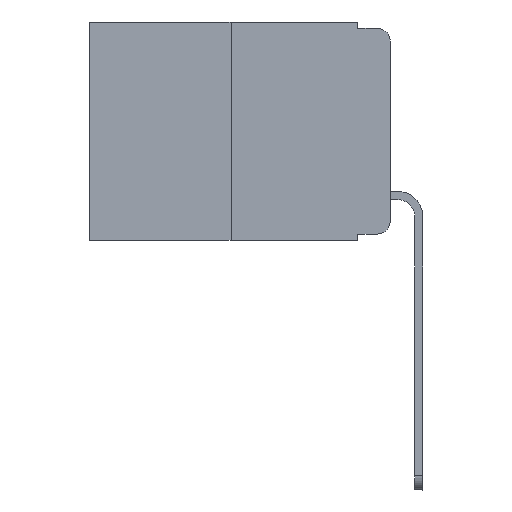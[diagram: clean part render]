
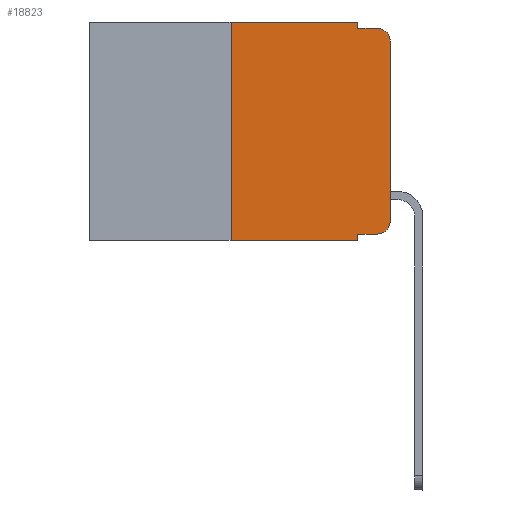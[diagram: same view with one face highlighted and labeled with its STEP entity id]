
A CAD part, left-side view. The second image highlights one B-rep face of the part: STEP entity #18823.
In plain terms, the highlighted planar face has unit normal (-1, 0, 0).
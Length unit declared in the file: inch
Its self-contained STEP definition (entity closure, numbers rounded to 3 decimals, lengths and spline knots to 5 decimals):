
#326 = EDGE_CURVE ( 'NONE', #14275, #2661, #22049, .T. ) ;
#783 = LINE ( 'NONE', #25401, #3292 ) ;
#1665 = VECTOR ( 'NONE', #16096, 39.37008 ) ;
#2250 = VECTOR ( 'NONE', #9095, 39.37008 ) ;
#2661 = VERTEX_POINT ( 'NONE', #17127 ) ;
#2748 = CARTESIAN_POINT ( 'NONE',  ( 0., 0.25, 0. ) ) ;
#2987 = ORIENTED_EDGE ( 'NONE', *, *, #16214, .T. ) ;
#3099 = ORIENTED_EDGE ( 'NONE', *, *, #326, .F. ) ;
#3292 = VECTOR ( 'NONE', #9144, 39.37008 ) ;
#3828 = EDGE_CURVE ( 'NONE', #10233, #14029, #17336, .T. ) ;
#3970 = CARTESIAN_POINT ( 'NONE',  ( 0., 0.02, -0.03 ) ) ;
#4244 = VECTOR ( 'NONE', #16767, 39.37008 ) ;
#4571 = LINE ( 'NONE', #13319, #2250 ) ;
#4583 = DIRECTION ( 'NONE',  ( 1., 0., 0. ) ) ;
#4977 = VERTEX_POINT ( 'NONE', #24141 ) ;
#5129 = DIRECTION ( 'NONE',  ( 0., 0., 1. ) ) ;
#5194 = CIRCLE ( 'NONE', #20494, 0.02 ) ;
#6585 = VERTEX_POINT ( 'NONE', #20843 ) ;
#6778 = CARTESIAN_POINT ( 'NONE',  ( 0., 0.25, 0. ) ) ;
#6905 = CARTESIAN_POINT ( 'NONE',  ( 0., 0.473, 0. ) ) ;
#6907 = LINE ( 'NONE', #6778, #19446 ) ;
#7227 = EDGE_LOOP ( 'NONE', ( #26319, #15640, #26040, #3099, #22942, #13227, #10855, #12541, #2987, #14217 ) ) ;
#7603 = DIRECTION ( 'NONE',  ( 0., 0., -1. ) ) ;
#7754 = CARTESIAN_POINT ( 'NONE',  ( 0., 0., 0. ) ) ;
#8421 = CARTESIAN_POINT ( 'NONE',  ( 0., 0.473, -0.343 ) ) ;
#8543 = VECTOR ( 'NONE', #18561, 39.37008 ) ;
#8771 = CARTESIAN_POINT ( 'NONE',  ( 0., 0.051, 0. ) ) ;
#9095 = DIRECTION ( 'NONE',  ( 0., 0., -1. ) ) ;
#9144 = DIRECTION ( 'NONE',  ( 0., -1., 0. ) ) ;
#9591 = DIRECTION ( 'NONE',  ( 0., 0., -1. ) ) ;
#10212 = VERTEX_POINT ( 'NONE', #18459 ) ;
#10233 = VERTEX_POINT ( 'NONE', #26485 ) ;
#10532 = EDGE_CURVE ( 'NONE', #11421, #14275, #783, .T. ) ;
#10855 = ORIENTED_EDGE ( 'NONE', *, *, #17451, .T. ) ;
#10872 = PLANE ( 'NONE',  #22212 ) ;
#11386 = CARTESIAN_POINT ( 'NONE',  ( 0., 0.051, 0. ) ) ;
#11421 = VERTEX_POINT ( 'NONE', #2748 ) ;
#11928 = EDGE_CURVE ( 'NONE', #14029, #21160, #26198, .T. ) ;
#12328 = DIRECTION ( 'NONE',  ( -1., 0., 0. ) ) ;
#12541 = ORIENTED_EDGE ( 'NONE', *, *, #23210, .F. ) ;
#12907 = LINE ( 'NONE', #25079, #26663 ) ;
#13227 = ORIENTED_EDGE ( 'NONE', *, *, #13306, .F. ) ;
#13306 = EDGE_CURVE ( 'NONE', #4977, #11421, #6907, .T. ) ;
#13319 = CARTESIAN_POINT ( 'NONE',  ( 0., 0.051, 0. ) ) ;
#13845 = VERTEX_POINT ( 'NONE', #19761 ) ;
#14029 = VERTEX_POINT ( 'NONE', #22983 ) ;
#14145 = DIRECTION ( 'NONE',  ( -1., 0., 0. ) ) ;
#14217 = ORIENTED_EDGE ( 'NONE', *, *, #3828, .T. ) ;
#14275 = VERTEX_POINT ( 'NONE', #8771 ) ;
#14612 = VECTOR ( 'NONE', #9591, 39.37008 ) ;
#15640 = ORIENTED_EDGE ( 'NONE', *, *, #19545, .T. ) ;
#16096 = DIRECTION ( 'NONE',  ( 0., 0., 1. ) ) ;
#16214 = EDGE_CURVE ( 'NONE', #6585, #10233, #26597, .T. ) ;
#16767 = DIRECTION ( 'NONE',  ( 0., -1., 0. ) ) ;
#17127 = CARTESIAN_POINT ( 'NONE',  ( 0., 0.051, -0.01 ) ) ;
#17336 = CIRCLE ( 'NONE', #24294, 0.02 ) ;
#17451 = EDGE_CURVE ( 'NONE', #4977, #13845, #18835, .T. ) ;
#18459 = CARTESIAN_POINT ( 'NONE',  ( 0., 0.02, -0.01 ) ) ;
#18542 = DIRECTION ( 'NONE',  ( 0., -1., 0. ) ) ;
#18561 = DIRECTION ( 'NONE',  ( 0., -1., 0. ) ) ;
#18823 = ADVANCED_FACE ( 'NONE', ( #25760 ), #10872, .F. ) ;
#18835 = LINE ( 'NONE', #8421, #4244 ) ;
#19446 = VECTOR ( 'NONE', #5129, 39.37008 ) ;
#19545 = EDGE_CURVE ( 'NONE', #21160, #10212, #5194, .T. ) ;
#19761 = CARTESIAN_POINT ( 'NONE',  ( 0., 0.051, -0.343 ) ) ;
#20388 = CARTESIAN_POINT ( 'NONE',  ( 0., 0., -0.03 ) ) ;
#20494 = AXIS2_PLACEMENT_3D ( 'NONE', #3970, #12328, #20696 ) ;
#20696 = DIRECTION ( 'NONE',  ( 0., 0., -1. ) ) ;
#20843 = CARTESIAN_POINT ( 'NONE',  ( 0., 0.051, -0.333 ) ) ;
#21160 = VERTEX_POINT ( 'NONE', #20388 ) ;
#22049 = LINE ( 'NONE', #11386, #14612 ) ;
#22212 = AXIS2_PLACEMENT_3D ( 'NONE', #6905, #4583, #25494 ) ;
#22942 = ORIENTED_EDGE ( 'NONE', *, *, #10532, .F. ) ;
#22983 = CARTESIAN_POINT ( 'NONE',  ( 0., 0., -0.313 ) ) ;
#23068 = EDGE_CURVE ( 'NONE', #2661, #10212, #12907, .T. ) ;
#23210 = EDGE_CURVE ( 'NONE', #6585, #13845, #4571, .T. ) ;
#24141 = CARTESIAN_POINT ( 'NONE',  ( 0., 0.25, -0.343 ) ) ;
#24294 = AXIS2_PLACEMENT_3D ( 'NONE', #26300, #14145, #7603 ) ;
#24971 = CARTESIAN_POINT ( 'NONE',  ( 0., 0.051, -0.333 ) ) ;
#25079 = CARTESIAN_POINT ( 'NONE',  ( 0., 0.051, -0.01 ) ) ;
#25401 = CARTESIAN_POINT ( 'NONE',  ( 0., 0.473, 0. ) ) ;
#25494 = DIRECTION ( 'NONE',  ( 0., 0., -1. ) ) ;
#25760 = FACE_OUTER_BOUND ( 'NONE', #7227, .T. ) ;
#26040 = ORIENTED_EDGE ( 'NONE', *, *, #23068, .F. ) ;
#26198 = LINE ( 'NONE', #7754, #1665 ) ;
#26300 = CARTESIAN_POINT ( 'NONE',  ( 0., 0.02, -0.313 ) ) ;
#26319 = ORIENTED_EDGE ( 'NONE', *, *, #11928, .T. ) ;
#26485 = CARTESIAN_POINT ( 'NONE',  ( 0., 0.02, -0.333 ) ) ;
#26597 = LINE ( 'NONE', #24971, #8543 ) ;
#26663 = VECTOR ( 'NONE', #18542, 39.37008 ) ;
